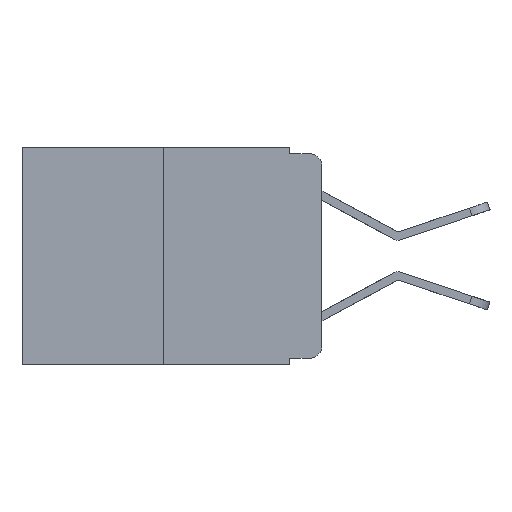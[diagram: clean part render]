
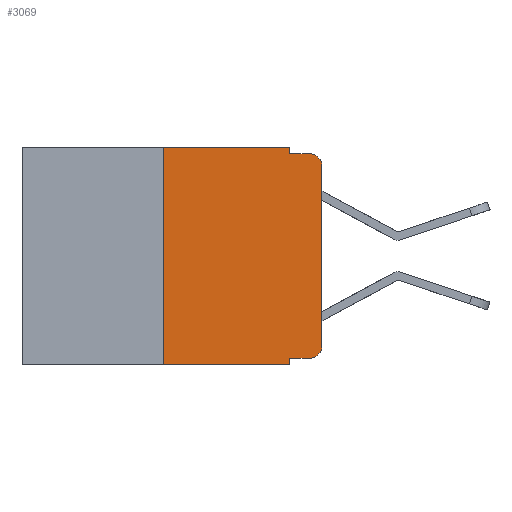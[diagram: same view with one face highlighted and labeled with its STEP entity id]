
A CAD part, left-side view. The second image highlights one B-rep face of the part: STEP entity #3069.
In plain terms, the highlighted planar face has unit normal (-1, 0, 0).
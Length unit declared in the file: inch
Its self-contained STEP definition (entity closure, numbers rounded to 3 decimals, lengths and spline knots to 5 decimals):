
#15 = VERTEX_POINT ( 'NONE', #4837 ) ;
#197 = VECTOR ( 'NONE', #9397, 39.37008 ) ;
#237 = CARTESIAN_POINT ( 'NONE',  ( 0., 0., 0. ) ) ;
#305 = DIRECTION ( 'NONE',  ( 0., 0., 1. ) ) ;
#907 = DIRECTION ( 'NONE',  ( 0., 0., 1. ) ) ;
#1014 = LINE ( 'NONE', #9999, #9565 ) ;
#1120 = VECTOR ( 'NONE', #305, 39.37008 ) ;
#1241 = ORIENTED_EDGE ( 'NONE', *, *, #12098, .F. ) ;
#1437 = EDGE_CURVE ( 'NONE', #17085, #8374, #18732, .T. ) ;
#1491 = VERTEX_POINT ( 'NONE', #10497 ) ;
#1768 = ORIENTED_EDGE ( 'NONE', *, *, #6839, .F. ) ;
#2539 = EDGE_CURVE ( 'NONE', #2744, #17085, #1014, .T. ) ;
#2744 = VERTEX_POINT ( 'NONE', #8939 ) ;
#2746 = CIRCLE ( 'NONE', #17454, 0.02 ) ;
#3069 = ADVANCED_FACE ( 'NONE', ( #14606 ), #15893, .F. ) ;
#3301 = ORIENTED_EDGE ( 'NONE', *, *, #9511, .T. ) ;
#3434 = CARTESIAN_POINT ( 'NONE',  ( 0., 0.051, -0.343 ) ) ;
#3608 = EDGE_CURVE ( 'NONE', #2744, #11442, #3623, .T. ) ;
#3623 = LINE ( 'NONE', #14159, #11558 ) ;
#4686 = LINE ( 'NONE', #7630, #8395 ) ;
#4837 = CARTESIAN_POINT ( 'NONE',  ( 0., 0.25, -0.343 ) ) ;
#4841 = ORIENTED_EDGE ( 'NONE', *, *, #1437, .T. ) ;
#4941 = CARTESIAN_POINT ( 'NONE',  ( 0., 0.051, 0. ) ) ;
#4993 = CARTESIAN_POINT ( 'NONE',  ( 0., 0.051, -0.01 ) ) ;
#5080 = ORIENTED_EDGE ( 'NONE', *, *, #16186, .T. ) ;
#5800 = EDGE_CURVE ( 'NONE', #15, #11470, #20075, .T. ) ;
#6614 = EDGE_CURVE ( 'NONE', #11470, #11387, #8771, .T. ) ;
#6670 = DIRECTION ( 'NONE',  ( 0., 0., -1. ) ) ;
#6839 = EDGE_CURVE ( 'NONE', #11387, #14224, #16703, .T. ) ;
#7055 = AXIS2_PLACEMENT_3D ( 'NONE', #19494, #19453, #19367 ) ;
#7560 = ORIENTED_EDGE ( 'NONE', *, *, #3608, .F. ) ;
#7630 = CARTESIAN_POINT ( 'NONE',  ( 0., 0.473, -0.343 ) ) ;
#8234 = DIRECTION ( 'NONE',  ( -1., 0., 0. ) ) ;
#8374 = VERTEX_POINT ( 'NONE', #18862 ) ;
#8395 = VECTOR ( 'NONE', #19909, 39.37008 ) ;
#8771 = LINE ( 'NONE', #15526, #197 ) ;
#8939 = CARTESIAN_POINT ( 'NONE',  ( 0., 0.051, -0.333 ) ) ;
#9283 = ORIENTED_EDGE ( 'NONE', *, *, #14170, .T. ) ;
#9397 = DIRECTION ( 'NONE',  ( 0., -1., 0. ) ) ;
#9511 = EDGE_CURVE ( 'NONE', #15, #11442, #4686, .T. ) ;
#9565 = VECTOR ( 'NONE', #19148, 39.37008 ) ;
#9666 = LINE ( 'NONE', #237, #1120 ) ;
#9849 = CARTESIAN_POINT ( 'NONE',  ( 0., 0.25, 0. ) ) ;
#9978 = CARTESIAN_POINT ( 'NONE',  ( 0., 0.02, -0.333 ) ) ;
#9999 = CARTESIAN_POINT ( 'NONE',  ( 0., 0.051, -0.333 ) ) ;
#10485 = EDGE_LOOP ( 'NONE', ( #5080, #9283, #1241, #1768, #14378, #14832, #3301, #7560, #12224, #4841 ) ) ;
#10497 = CARTESIAN_POINT ( 'NONE',  ( 0., 0., -0.03 ) ) ;
#10525 = CARTESIAN_POINT ( 'NONE',  ( 0., 0.25, 0. ) ) ;
#11387 = VERTEX_POINT ( 'NONE', #4941 ) ;
#11442 = VERTEX_POINT ( 'NONE', #3434 ) ;
#11470 = VERTEX_POINT ( 'NONE', #9849 ) ;
#11516 = LINE ( 'NONE', #4993, #19604 ) ;
#11558 = VECTOR ( 'NONE', #17193, 39.37008 ) ;
#12098 = EDGE_CURVE ( 'NONE', #14224, #13236, #11516, .T. ) ;
#12224 = ORIENTED_EDGE ( 'NONE', *, *, #2539, .T. ) ;
#12896 = CARTESIAN_POINT ( 'NONE',  ( 0., 0.473, 0. ) ) ;
#12987 = DIRECTION ( 'NONE',  ( 0., 0., -1. ) ) ;
#13144 = VECTOR ( 'NONE', #12987, 39.37008 ) ;
#13236 = VERTEX_POINT ( 'NONE', #14181 ) ;
#14159 = CARTESIAN_POINT ( 'NONE',  ( 0., 0.051, 0. ) ) ;
#14170 = EDGE_CURVE ( 'NONE', #1491, #13236, #2746, .T. ) ;
#14181 = CARTESIAN_POINT ( 'NONE',  ( 0., 0.02, -0.01 ) ) ;
#14224 = VERTEX_POINT ( 'NONE', #17517 ) ;
#14360 = DIRECTION ( 'NONE',  ( 0., -1., 0. ) ) ;
#14378 = ORIENTED_EDGE ( 'NONE', *, *, #6614, .F. ) ;
#14606 = FACE_OUTER_BOUND ( 'NONE', #10485, .T. ) ;
#14832 = ORIENTED_EDGE ( 'NONE', *, *, #5800, .F. ) ;
#15526 = CARTESIAN_POINT ( 'NONE',  ( 0., 0.473, 0. ) ) ;
#15893 = PLANE ( 'NONE',  #18597 ) ;
#15957 = DIRECTION ( 'NONE',  ( 1., 0., 0. ) ) ;
#16047 = CARTESIAN_POINT ( 'NONE',  ( 0., 0.051, 0. ) ) ;
#16186 = EDGE_CURVE ( 'NONE', #8374, #1491, #9666, .T. ) ;
#16703 = LINE ( 'NONE', #16047, #13144 ) ;
#17085 = VERTEX_POINT ( 'NONE', #9978 ) ;
#17193 = DIRECTION ( 'NONE',  ( 0., 0., -1. ) ) ;
#17454 = AXIS2_PLACEMENT_3D ( 'NONE', #17461, #8234, #18985 ) ;
#17461 = CARTESIAN_POINT ( 'NONE',  ( 0., 0.02, -0.03 ) ) ;
#17517 = CARTESIAN_POINT ( 'NONE',  ( 0., 0.051, -0.01 ) ) ;
#18597 = AXIS2_PLACEMENT_3D ( 'NONE', #12896, #15957, #6670 ) ;
#18732 = CIRCLE ( 'NONE', #7055, 0.02 ) ;
#18862 = CARTESIAN_POINT ( 'NONE',  ( 0., 0., -0.313 ) ) ;
#18985 = DIRECTION ( 'NONE',  ( 0., 0., -1. ) ) ;
#19148 = DIRECTION ( 'NONE',  ( 0., -1., 0. ) ) ;
#19367 = DIRECTION ( 'NONE',  ( 0., 0., -1. ) ) ;
#19453 = DIRECTION ( 'NONE',  ( -1., 0., 0. ) ) ;
#19494 = CARTESIAN_POINT ( 'NONE',  ( 0., 0.02, -0.313 ) ) ;
#19594 = VECTOR ( 'NONE', #907, 39.37008 ) ;
#19604 = VECTOR ( 'NONE', #14360, 39.37008 ) ;
#19909 = DIRECTION ( 'NONE',  ( 0., -1., 0. ) ) ;
#20075 = LINE ( 'NONE', #10525, #19594 ) ;
